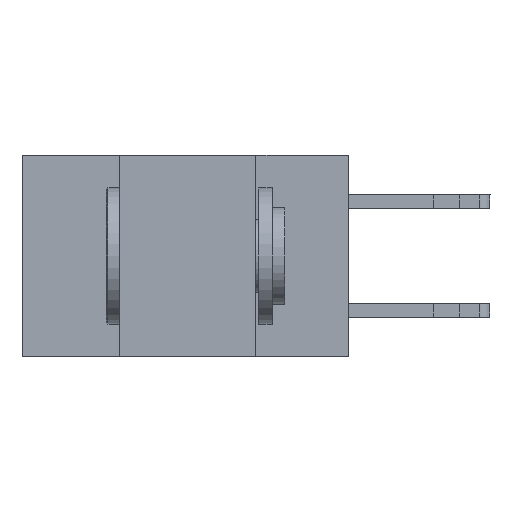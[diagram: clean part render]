
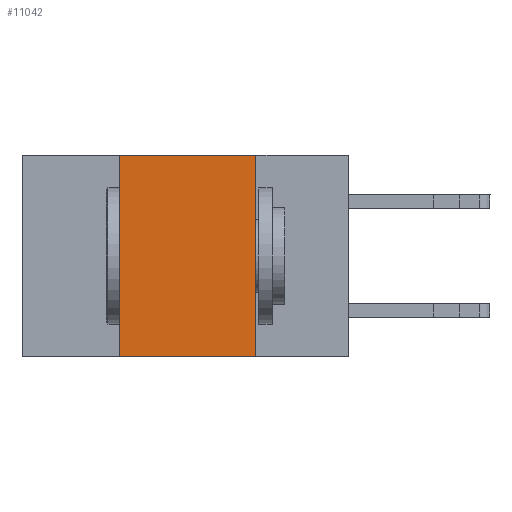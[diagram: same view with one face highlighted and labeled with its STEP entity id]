
A CAD part, left-side view. The second image highlights one B-rep face of the part: STEP entity #11042.
In plain terms, the highlighted planar face has unit normal (-1, 0, 0).
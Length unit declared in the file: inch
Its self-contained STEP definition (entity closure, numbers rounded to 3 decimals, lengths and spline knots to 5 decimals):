
#140 = ORIENTED_EDGE ( 'NONE', *, *, #9864, .F. ) ;
#715 = EDGE_CURVE ( 'NONE', #828, #19058, #5516, .T. ) ;
#804 = CARTESIAN_POINT ( 'NONE',  ( 0., 0.17, 0. ) ) ;
#828 = VERTEX_POINT ( 'NONE', #9561 ) ;
#1287 = CARTESIAN_POINT ( 'NONE',  ( 0., 0.6, 0. ) ) ;
#1301 = VECTOR ( 'NONE', #6309, 39.37008 ) ;
#2132 = CARTESIAN_POINT ( 'NONE',  ( 0., 0.42, 0. ) ) ;
#3292 = CARTESIAN_POINT ( 'NONE',  ( 0., 0.6, -0.37 ) ) ;
#4292 = CARTESIAN_POINT ( 'NONE',  ( 0., 0.6, 0. ) ) ;
#4352 = ORIENTED_EDGE ( 'NONE', *, *, #5631, .T. ) ;
#5223 = ORIENTED_EDGE ( 'NONE', *, *, #715, .F. ) ;
#5516 = LINE ( 'NONE', #804, #20668 ) ;
#5631 = EDGE_CURVE ( 'NONE', #10076, #19058, #18068, .T. ) ;
#5674 = VECTOR ( 'NONE', #7568, 39.37008 ) ;
#5994 = DIRECTION ( 'NONE',  ( 1., 0., 0. ) ) ;
#6309 = DIRECTION ( 'NONE',  ( 0., -1., 0. ) ) ;
#6673 = EDGE_CURVE ( 'NONE', #10076, #14297, #15230, .T. ) ;
#6798 = VECTOR ( 'NONE', #18161, 39.37008 ) ;
#7423 = DIRECTION ( 'NONE',  ( 0., 0., -1. ) ) ;
#7568 = DIRECTION ( 'NONE',  ( 0., 0., 1. ) ) ;
#8741 = CARTESIAN_POINT ( 'NONE',  ( 0., 0.42, 0. ) ) ;
#9561 = CARTESIAN_POINT ( 'NONE',  ( 0., 0.17, 0. ) ) ;
#9715 = LINE ( 'NONE', #1287, #1301 ) ;
#9864 = EDGE_CURVE ( 'NONE', #14297, #828, #9715, .T. ) ;
#10066 = AXIS2_PLACEMENT_3D ( 'NONE', #4292, #5994, #17161 ) ;
#10076 = VERTEX_POINT ( 'NONE', #10557 ) ;
#10557 = CARTESIAN_POINT ( 'NONE',  ( 0., 0.42, -0.37 ) ) ;
#11042 = ADVANCED_FACE ( 'NONE', ( #20561 ), #20349, .F. ) ;
#11523 = CARTESIAN_POINT ( 'NONE',  ( 0., 0.17, -0.37 ) ) ;
#14297 = VERTEX_POINT ( 'NONE', #2132 ) ;
#15230 = LINE ( 'NONE', #8741, #5674 ) ;
#16952 = ORIENTED_EDGE ( 'NONE', *, *, #6673, .F. ) ;
#17161 = DIRECTION ( 'NONE',  ( 0., 0., -1. ) ) ;
#18068 = LINE ( 'NONE', #3292, #6798 ) ;
#18161 = DIRECTION ( 'NONE',  ( 0., -1., 0. ) ) ;
#18853 = EDGE_LOOP ( 'NONE', ( #5223, #140, #16952, #4352 ) ) ;
#19058 = VERTEX_POINT ( 'NONE', #11523 ) ;
#20349 = PLANE ( 'NONE',  #10066 ) ;
#20561 = FACE_OUTER_BOUND ( 'NONE', #18853, .T. ) ;
#20668 = VECTOR ( 'NONE', #7423, 39.37008 ) ;
